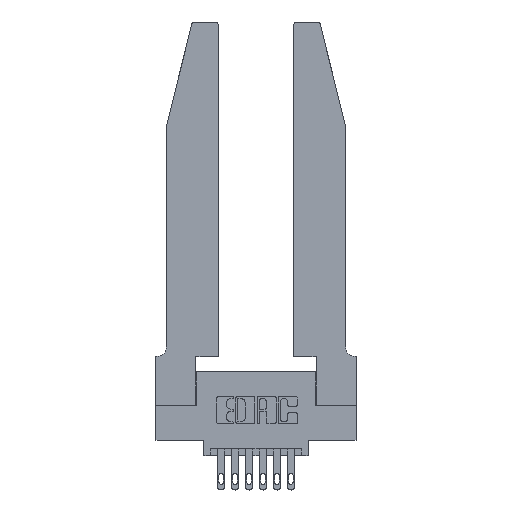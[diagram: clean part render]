
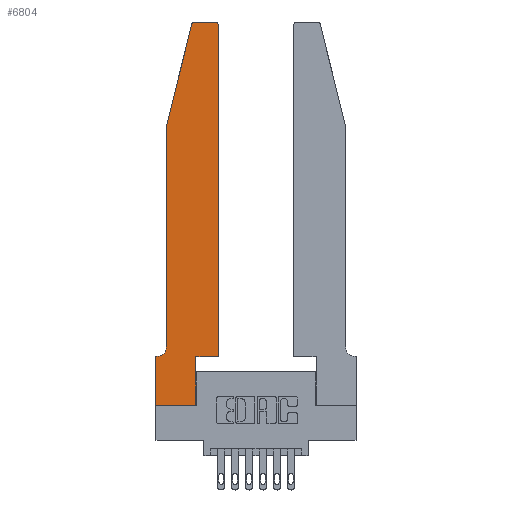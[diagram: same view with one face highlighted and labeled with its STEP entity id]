
A CAD part, top view. The second image highlights one B-rep face of the part: STEP entity #6804.
In plain terms, the highlighted planar face has unit normal (0, 0, 1).
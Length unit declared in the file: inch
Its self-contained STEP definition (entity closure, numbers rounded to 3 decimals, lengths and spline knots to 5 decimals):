
#40 = CARTESIAN_POINT ( 'NONE',  ( 0.4505, 0.35, 0.37 ) ) ;
#211 = VERTEX_POINT ( 'NONE', #4712 ) ;
#259 = CARTESIAN_POINT ( 'NONE',  ( 0.2605, 2.75, 0.37 ) ) ;
#320 = CARTESIAN_POINT ( 'NONE',  ( 0.25487, 2.72718, 0.37 ) ) ;
#399 = LINE ( 'NONE', #836, #11928 ) ;
#524 = VECTOR ( 'NONE', #9043, 39.37008 ) ;
#531 = CARTESIAN_POINT ( 'NONE',  ( 0.4505, 0.35, 0.37 ) ) ;
#597 = EDGE_CURVE ( 'NONE', #1608, #10250, #8750, .T. ) ;
#610 = DIRECTION ( 'NONE',  ( 1., 0., 0. ) ) ;
#619 = EDGE_LOOP ( 'NONE', ( #4251, #11925, #1094, #5144, #10607, #13399, #11325, #5104, #14201, #2679, #8145, #2902 ) ) ;
#836 = CARTESIAN_POINT ( 'NONE',  ( 0.0755, 2., 0.37 ) ) ;
#930 = CIRCLE ( 'NONE', #11056, 0.03 ) ;
#1094 = ORIENTED_EDGE ( 'NONE', *, *, #7195, .T. ) ;
#1608 = VERTEX_POINT ( 'NONE', #4351 ) ;
#1757 = CARTESIAN_POINT ( 'NONE',  ( 0.0055, 0.42, 0.37 ) ) ;
#1931 = EDGE_CURVE ( 'NONE', #13308, #13412, #3998, .T. ) ;
#2043 = EDGE_CURVE ( 'NONE', #10250, #3993, #10460, .T. ) ;
#2070 = LINE ( 'NONE', #13997, #11858 ) ;
#2131 = EDGE_CURVE ( 'NONE', #3993, #5385, #2070, .T. ) ;
#2254 = VECTOR ( 'NONE', #3895, 39.37008 ) ;
#2321 = DIRECTION ( 'NONE',  ( 1., 0., 0. ) ) ;
#2363 = CARTESIAN_POINT ( 'NONE',  ( 0., 0.35, 0.37 ) ) ;
#2417 = CARTESIAN_POINT ( 'NONE',  ( 0.0755, 2., 0.37 ) ) ;
#2679 = ORIENTED_EDGE ( 'NONE', *, *, #1931, .T. ) ;
#2813 = EDGE_CURVE ( 'NONE', #9094, #13308, #7624, .T. ) ;
#2875 = FACE_OUTER_BOUND ( 'NONE', #619, .T. ) ;
#2902 = ORIENTED_EDGE ( 'NONE', *, *, #14080, .T. ) ;
#3061 = CARTESIAN_POINT ( 'NONE',  ( 0.2865, 0.35, 0.37 ) ) ;
#3535 = DIRECTION ( 'NONE',  ( -1., 0., 0. ) ) ;
#3895 = DIRECTION ( 'NONE',  ( 1., 0., 0. ) ) ;
#3993 = VERTEX_POINT ( 'NONE', #2363 ) ;
#3998 = LINE ( 'NONE', #531, #2254 ) ;
#4251 = ORIENTED_EDGE ( 'NONE', *, *, #14264, .T. ) ;
#4351 = CARTESIAN_POINT ( 'NONE',  ( 0.0755, 0.42, 0.37 ) ) ;
#4611 = VERTEX_POINT ( 'NONE', #13642 ) ;
#4694 = DIRECTION ( 'NONE',  ( 0., 0., 1. ) ) ;
#4707 = VECTOR ( 'NONE', #6131, 39.37008 ) ;
#4712 = CARTESIAN_POINT ( 'NONE',  ( 0.4505, 2.72, 0.37 ) ) ;
#5100 = CIRCLE ( 'NONE', #12042, 0.03 ) ;
#5104 = ORIENTED_EDGE ( 'NONE', *, *, #5861, .T. ) ;
#5144 = ORIENTED_EDGE ( 'NONE', *, *, #8772, .T. ) ;
#5274 = CARTESIAN_POINT ( 'NONE',  ( 0.0755, 2., 0.37 ) ) ;
#5385 = VERTEX_POINT ( 'NONE', #7129 ) ;
#5662 = CARTESIAN_POINT ( 'NONE',  ( 0.284, 2.75, 0.37 ) ) ;
#5815 = DIRECTION ( 'NONE',  ( 1., 0., 0. ) ) ;
#5861 = EDGE_CURVE ( 'NONE', #5385, #9094, #10076, .T. ) ;
#6062 = VECTOR ( 'NONE', #610, 39.37008 ) ;
#6131 = DIRECTION ( 'NONE',  ( -1., 0., 0. ) ) ;
#6317 = DIRECTION ( 'NONE',  ( 0., -1., 0. ) ) ;
#6554 = DIRECTION ( 'NONE',  ( 1., 0., 0. ) ) ;
#6804 = ADVANCED_FACE ( 'NONE', ( #2875 ), #8575, .T. ) ;
#7129 = CARTESIAN_POINT ( 'NONE',  ( 0., 0., 0.37 ) ) ;
#7195 = EDGE_CURVE ( 'NONE', #13831, #10616, #9677, .T. ) ;
#7412 = DIRECTION ( 'NONE',  ( 0., 0., -1. ) ) ;
#7624 = LINE ( 'NONE', #3061, #10253 ) ;
#7806 = VERTEX_POINT ( 'NONE', #5662 ) ;
#8013 = CARTESIAN_POINT ( 'NONE',  ( 0.284, 2.72, 0.37 ) ) ;
#8145 = ORIENTED_EDGE ( 'NONE', *, *, #11202, .T. ) ;
#8575 = PLANE ( 'NONE',  #9669 ) ;
#8627 = VECTOR ( 'NONE', #12174, 39.37008 ) ;
#8659 = CARTESIAN_POINT ( 'NONE',  ( 0.4205, 2.72, 0.37 ) ) ;
#8750 = CIRCLE ( 'NONE', #9008, 0.07 ) ;
#8772 = EDGE_CURVE ( 'NONE', #10616, #1608, #399, .T. ) ;
#9008 = AXIS2_PLACEMENT_3D ( 'NONE', #1757, #7412, #12975 ) ;
#9043 = DIRECTION ( 'NONE',  ( 0., 1., 0. ) ) ;
#9094 = VERTEX_POINT ( 'NONE', #9193 ) ;
#9193 = CARTESIAN_POINT ( 'NONE',  ( 0.2865, 0., 0.37 ) ) ;
#9208 = EDGE_CURVE ( 'NONE', #7806, #13831, #5100, .T. ) ;
#9669 = AXIS2_PLACEMENT_3D ( 'NONE', #10803, #11936, #6554 ) ;
#9677 = LINE ( 'NONE', #5274, #8627 ) ;
#9770 = LINE ( 'NONE', #40, #524 ) ;
#10076 = LINE ( 'NONE', #10612, #6062 ) ;
#10199 = LINE ( 'NONE', #259, #10552 ) ;
#10250 = VERTEX_POINT ( 'NONE', #13078 ) ;
#10253 = VECTOR ( 'NONE', #13052, 39.37008 ) ;
#10460 = LINE ( 'NONE', #12725, #4707 ) ;
#10552 = VECTOR ( 'NONE', #3535, 39.37008 ) ;
#10607 = ORIENTED_EDGE ( 'NONE', *, *, #597, .T. ) ;
#10612 = CARTESIAN_POINT ( 'NONE',  ( 0., 0., 0.37 ) ) ;
#10616 = VERTEX_POINT ( 'NONE', #2417 ) ;
#10803 = CARTESIAN_POINT ( 'NONE',  ( 0., 0.35, 0.37 ) ) ;
#11056 = AXIS2_PLACEMENT_3D ( 'NONE', #8659, #12801, #2321 ) ;
#11202 = EDGE_CURVE ( 'NONE', #13412, #211, #9770, .T. ) ;
#11325 = ORIENTED_EDGE ( 'NONE', *, *, #2131, .T. ) ;
#11858 = VECTOR ( 'NONE', #6317, 39.37008 ) ;
#11925 = ORIENTED_EDGE ( 'NONE', *, *, #9208, .T. ) ;
#11928 = VECTOR ( 'NONE', #12054, 39.37008 ) ;
#11936 = DIRECTION ( 'NONE',  ( 0., 0., 1. ) ) ;
#12042 = AXIS2_PLACEMENT_3D ( 'NONE', #8013, #4694, #5815 ) ;
#12054 = DIRECTION ( 'NONE',  ( 0., -1., 0. ) ) ;
#12174 = DIRECTION ( 'NONE',  ( -0.239, -0.971, 0. ) ) ;
#12463 = CARTESIAN_POINT ( 'NONE',  ( 0.2865, 0.35, 0.37 ) ) ;
#12725 = CARTESIAN_POINT ( 'NONE',  ( 0.0755, 0.35, 0.37 ) ) ;
#12801 = DIRECTION ( 'NONE',  ( 0., 0., 1. ) ) ;
#12975 = DIRECTION ( 'NONE',  ( -1., 0., 0. ) ) ;
#13052 = DIRECTION ( 'NONE',  ( 0., 1., 0. ) ) ;
#13078 = CARTESIAN_POINT ( 'NONE',  ( 0.0055, 0.35, 0.37 ) ) ;
#13308 = VERTEX_POINT ( 'NONE', #12463 ) ;
#13399 = ORIENTED_EDGE ( 'NONE', *, *, #2043, .T. ) ;
#13412 = VERTEX_POINT ( 'NONE', #13821 ) ;
#13642 = CARTESIAN_POINT ( 'NONE',  ( 0.4205, 2.75, 0.37 ) ) ;
#13821 = CARTESIAN_POINT ( 'NONE',  ( 0.4505, 0.35, 0.37 ) ) ;
#13831 = VERTEX_POINT ( 'NONE', #320 ) ;
#13997 = CARTESIAN_POINT ( 'NONE',  ( 0., 0., 0.37 ) ) ;
#14080 = EDGE_CURVE ( 'NONE', #211, #4611, #930, .T. ) ;
#14201 = ORIENTED_EDGE ( 'NONE', *, *, #2813, .T. ) ;
#14264 = EDGE_CURVE ( 'NONE', #4611, #7806, #10199, .T. ) ;
